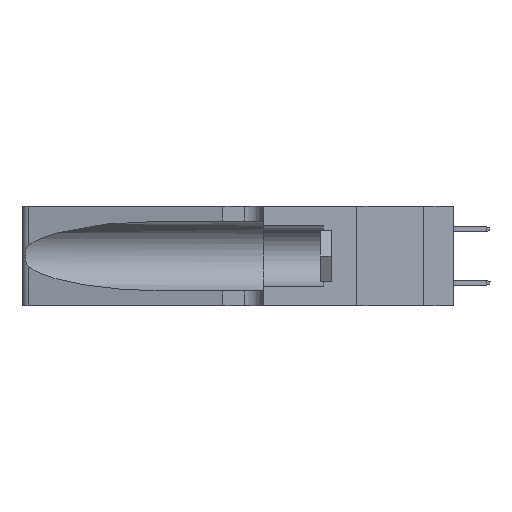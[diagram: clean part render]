
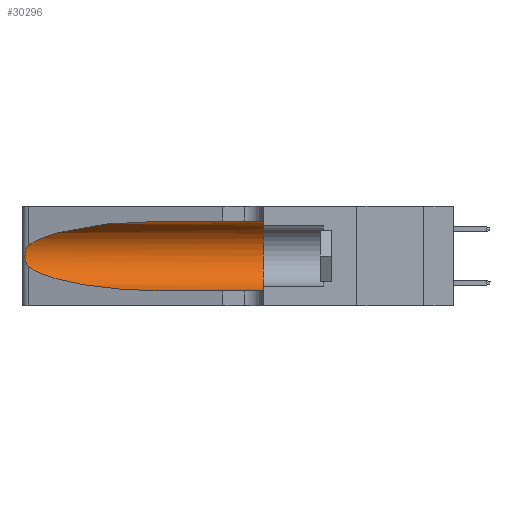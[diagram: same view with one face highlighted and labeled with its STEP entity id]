
A CAD part, left-side view. The second image highlights one B-rep face of the part: STEP entity #30296.
In plain terms, the highlighted cylindrical face has radius 3.308 mm (diameter 6.617 mm), a partial arc.
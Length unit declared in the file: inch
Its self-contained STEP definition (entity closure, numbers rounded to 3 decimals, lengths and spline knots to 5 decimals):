
#797 = CARTESIAN_POINT ( 'NONE',  ( 0.25487, 1.22718, 0.22369 ) ) ;
#973 = CARTESIAN_POINT ( 'NONE',  ( 0.25555, 1.22993, 0.14849 ) ) ;
#3283 = LINE ( 'NONE', #14025, #14626 ) ;
#4060 = CARTESIAN_POINT ( 'NONE',  ( 0.1305, 0.35, 0.185 ) ) ;
#5590 = VERTEX_POINT ( 'NONE', #30974 ) ;
#6245 = CARTESIAN_POINT ( 'NONE',  ( 0.25856, 1.23593, 0.16098 ) ) ;
#6310 = CARTESIAN_POINT ( 'NONE',  ( 0.1305, 0.35, 0.05475 ) ) ;
#6538 = DIRECTION ( 'NONE',  ( 0., 0., 1. ) ) ;
#6985 = CARTESIAN_POINT ( 'NONE',  ( 0.2373, 1.15595, 0.28018 ) ) ;
#8495 = ORIENTED_EDGE ( 'NONE', *, *, #9695, .T. ) ;
#8837 = CARTESIAN_POINT ( 'NONE',  ( 0.1305, 1.61858, 0.185 ) ) ;
#8842 = EDGE_CURVE ( 'NONE', #9619, #25954, #18978, .T. ) ;
#8907 = CARTESIAN_POINT ( 'NONE',  ( 0.26075, 1.23896, 0.19203 ) ) ;
#9387 =( BOUNDED_CURVE ( )  B_SPLINE_CURVE ( 3, ( #9620, #25073, #6985, #19993 ),
 .UNSPECIFIED., .F., .T. ) 
 B_SPLINE_CURVE_WITH_KNOTS ( ( 4, 4 ),
 ( 1.5708, 2.84003 ),
 .UNSPECIFIED. ) 
 CURVE ( )  GEOMETRIC_REPRESENTATION_ITEM ( )  RATIONAL_B_SPLINE_CURVE ( ( 1., 0.87, 0.87, 1. ) ) 
 REPRESENTATION_ITEM ( '' )  );
#9436 = ORIENTED_EDGE ( 'NONE', *, *, #26937, .F. ) ;
#9619 = VERTEX_POINT ( 'NONE', #24623 ) ;
#9620 = CARTESIAN_POINT ( 'NONE',  ( 0.1305, 0.72297, 0.31525 ) ) ;
#9695 = EDGE_CURVE ( 'NONE', #24492, #33418, #15616, .T. ) ;
#10521 = EDGE_CURVE ( 'NONE', #33418, #18060, #3283, .T. ) ;
#11112 = CYLINDRICAL_SURFACE ( 'NONE', #29852, 0.13025 ) ;
#11155 = EDGE_CURVE ( 'NONE', #5590, #24492, #14115, .T. ) ;
#11528 = CARTESIAN_POINT ( 'NONE',  ( 0.25854, 1.2359, 0.20912 ) ) ;
#14025 = CARTESIAN_POINT ( 'NONE',  ( 0.1305, 1.61858, 0.05475 ) ) ;
#14115 = B_SPLINE_CURVE_WITH_KNOTS ( 'NONE', 3,
 ( #797, #22384, #22208, #14156, #11528, #32921, #8907, #19936, #33102, #6245, #27630, #25008, #973, #30464 ),
 .UNSPECIFIED., .F., .F.,
 ( 4, 2, 2, 2, 2, 2, 4 ),
 ( 0., 0.00027, 0.00053, 0.00107, 0.0016, 0.00187, 0.00214 ),
 .UNSPECIFIED. ) ;
#14156 = CARTESIAN_POINT ( 'NONE',  ( 0.25787, 1.23484, 0.2124 ) ) ;
#14427 = CARTESIAN_POINT ( 'NONE',  ( 0.25487, 1.22718, 0.14631 ) ) ;
#14483 = AXIS2_PLACEMENT_3D ( 'NONE', #4060, #23009, #6538 ) ;
#14626 = VECTOR ( 'NONE', #22074, 39.37008 ) ;
#14714 = ORIENTED_EDGE ( 'NONE', *, *, #29475, .T. ) ;
#15616 =( BOUNDED_CURVE ( )  B_SPLINE_CURVE ( 3, ( #19367, #22337, #27238, #24796 ),
 .UNSPECIFIED., .F., .T. ) 
 B_SPLINE_CURVE_WITH_KNOTS ( ( 4, 4 ),
 ( 3.44316, 4.71239 ),
 .UNSPECIFIED. ) 
 CURVE ( )  GEOMETRIC_REPRESENTATION_ITEM ( )  RATIONAL_B_SPLINE_CURVE ( ( 1., 0.87, 0.87, 1. ) ) 
 REPRESENTATION_ITEM ( '' )  );
#16700 = CARTESIAN_POINT ( 'NONE',  ( 0.1305, 1.61858, 0.31525 ) ) ;
#18060 = VERTEX_POINT ( 'NONE', #6310 ) ;
#18978 = LINE ( 'NONE', #16700, #24039 ) ;
#19367 = CARTESIAN_POINT ( 'NONE',  ( 0.25487, 1.22718, 0.14631 ) ) ;
#19428 = CARTESIAN_POINT ( 'NONE',  ( 0.1305, 0.35, 0.31525 ) ) ;
#19521 = DIRECTION ( 'NONE',  ( 0., -1., 0. ) ) ;
#19936 = CARTESIAN_POINT ( 'NONE',  ( 0.26075, 1.23896, 0.178 ) ) ;
#19993 = CARTESIAN_POINT ( 'NONE',  ( 0.25487, 1.22718, 0.22369 ) ) ;
#22074 = DIRECTION ( 'NONE',  ( 0., -1., 0. ) ) ;
#22142 = FACE_OUTER_BOUND ( 'NONE', #26475, .T. ) ;
#22208 = CARTESIAN_POINT ( 'NONE',  ( 0.25639, 1.23184, 0.21858 ) ) ;
#22337 = CARTESIAN_POINT ( 'NONE',  ( 0.2373, 1.15595, 0.08982 ) ) ;
#22384 = CARTESIAN_POINT ( 'NONE',  ( 0.25555, 1.22994, 0.2215 ) ) ;
#23009 = DIRECTION ( 'NONE',  ( 0., 1., 0. ) ) ;
#24039 = VECTOR ( 'NONE', #24754, 39.37008 ) ;
#24492 = VERTEX_POINT ( 'NONE', #14427 ) ;
#24623 = CARTESIAN_POINT ( 'NONE',  ( 0.1305, 0.72297, 0.31525 ) ) ;
#24754 = DIRECTION ( 'NONE',  ( 0., -1., 0. ) ) ;
#24796 = CARTESIAN_POINT ( 'NONE',  ( 0.1305, 0.72297, 0.05475 ) ) ;
#25008 = CARTESIAN_POINT ( 'NONE',  ( 0.25639, 1.23186, 0.15144 ) ) ;
#25073 = CARTESIAN_POINT ( 'NONE',  ( 0.18966, 0.96281, 0.31525 ) ) ;
#25479 = CARTESIAN_POINT ( 'NONE',  ( 0.1305, 0.72297, 0.05475 ) ) ;
#25954 = VERTEX_POINT ( 'NONE', #19428 ) ;
#26249 = ORIENTED_EDGE ( 'NONE', *, *, #11155, .T. ) ;
#26475 = EDGE_LOOP ( 'NONE', ( #14714, #26249, #8495, #28052, #9436, #29645 ) ) ;
#26937 = EDGE_CURVE ( 'NONE', #25954, #18060, #30155, .T. ) ;
#27238 = CARTESIAN_POINT ( 'NONE',  ( 0.18966, 0.96281, 0.05475 ) ) ;
#27630 = CARTESIAN_POINT ( 'NONE',  ( 0.25789, 1.23486, 0.15765 ) ) ;
#28052 = ORIENTED_EDGE ( 'NONE', *, *, #10521, .T. ) ;
#29475 = EDGE_CURVE ( 'NONE', #9619, #5590, #9387, .T. ) ;
#29645 = ORIENTED_EDGE ( 'NONE', *, *, #8842, .F. ) ;
#29852 = AXIS2_PLACEMENT_3D ( 'NONE', #8837, #19521, #30215 ) ;
#30155 = CIRCLE ( 'NONE', #14483, 0.13025 ) ;
#30215 = DIRECTION ( 'NONE',  ( 0., 0., -1. ) ) ;
#30296 = ADVANCED_FACE ( 'NONE', ( #22142 ), #11112, .F. ) ;
#30464 = CARTESIAN_POINT ( 'NONE',  ( 0.25487, 1.22718, 0.14631 ) ) ;
#30974 = CARTESIAN_POINT ( 'NONE',  ( 0.25487, 1.22718, 0.22369 ) ) ;
#32921 = CARTESIAN_POINT ( 'NONE',  ( 0.26018, 1.23835, 0.19895 ) ) ;
#33102 = CARTESIAN_POINT ( 'NONE',  ( 0.26017, 1.23833, 0.17102 ) ) ;
#33418 = VERTEX_POINT ( 'NONE', #25479 ) ;
